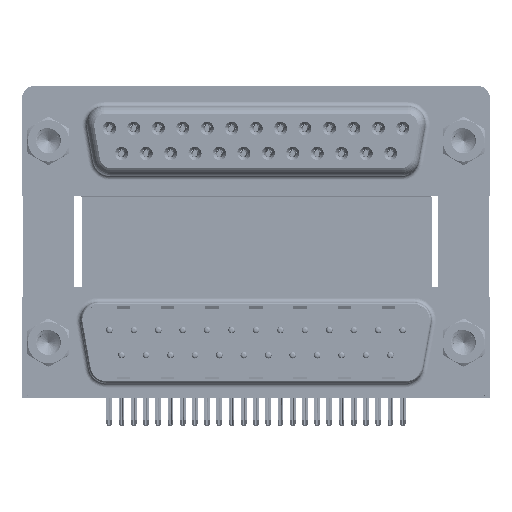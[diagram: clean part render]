
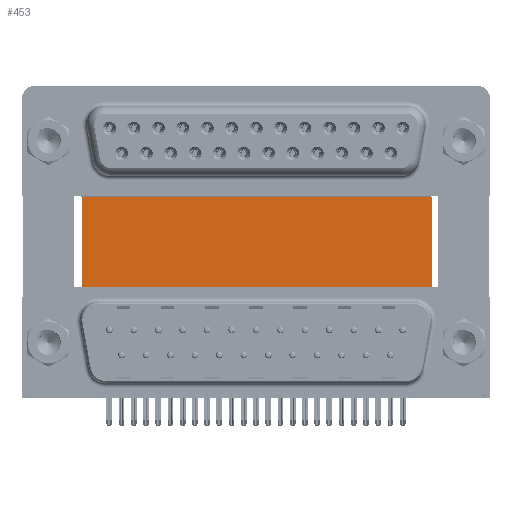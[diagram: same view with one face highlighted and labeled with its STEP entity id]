
A CAD part, top view. The second image highlights one B-rep face of the part: STEP entity #453.
In plain terms, the highlighted planar face has unit normal (0, 0, 1).
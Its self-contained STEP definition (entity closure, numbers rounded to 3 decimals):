
#93 = CARTESIAN_POINT ( 'NONE',  ( 3.79, 16.585, -12. ) ) ;
#308 = CARTESIAN_POINT ( 'NONE',  ( 43.43, 16.585, -12. ) ) ;
#453 = ADVANCED_FACE ( 'NONE', ( #34386 ), #1013, .F. ) ;
#1013 = PLANE ( 'NONE',  #60644 ) ;
#2868 = ORIENTED_EDGE ( 'NONE', *, *, #33222, .F. ) ;
#7323 = VERTEX_POINT ( 'NONE', #46095 ) ;
#10455 = DIRECTION ( 'NONE',  ( 0., 0., -1. ) ) ;
#12122 = VERTEX_POINT ( 'NONE', #308 ) ;
#15005 = LINE ( 'NONE', #48310, #37044 ) ;
#16457 = DIRECTION ( 'NONE',  ( 1., 0., 0. ) ) ;
#17712 = EDGE_CURVE ( 'NONE', #12122, #57683, #15005, .T. ) ;
#18959 = DIRECTION ( 'NONE',  ( 0., -1., 0. ) ) ;
#19459 = EDGE_CURVE ( 'NONE', #52430, #57683, #25617, .T. ) ;
#25617 = LINE ( 'NONE', #38851, #34199 ) ;
#25681 = VECTOR ( 'NONE', #16457, 1000. ) ;
#28084 = ORIENTED_EDGE ( 'NONE', *, *, #50141, .T. ) ;
#32612 = CARTESIAN_POINT ( 'NONE',  ( 3.79, -3.735, -12. ) ) ;
#33222 = EDGE_CURVE ( 'NONE', #7323, #12122, #40963, .T. ) ;
#33712 = LINE ( 'NONE', #53173, #38297 ) ;
#34198 = DIRECTION ( 'NONE',  ( 0., -1., 0. ) ) ;
#34199 = VECTOR ( 'NONE', #44788, 1000. ) ;
#34386 = FACE_OUTER_BOUND ( 'NONE', #46622, .T. ) ;
#37044 = VECTOR ( 'NONE', #34198, 1000. ) ;
#38297 = VECTOR ( 'NONE', #18959, 1000. ) ;
#38851 = CARTESIAN_POINT ( 'NONE',  ( 3.79, -3.735, -12. ) ) ;
#40963 = LINE ( 'NONE', #59491, #25681 ) ;
#44788 = DIRECTION ( 'NONE',  ( 1., 0., 0. ) ) ;
#46095 = CARTESIAN_POINT ( 'NONE',  ( 3.79, 16.585, -12. ) ) ;
#46622 = EDGE_LOOP ( 'NONE', ( #52943, #48992, #2868, #28084 ) ) ;
#48310 = CARTESIAN_POINT ( 'NONE',  ( 43.43, 16.585, -12. ) ) ;
#48992 = ORIENTED_EDGE ( 'NONE', *, *, #17712, .F. ) ;
#50141 = EDGE_CURVE ( 'NONE', #7323, #52430, #33712, .T. ) ;
#52430 = VERTEX_POINT ( 'NONE', #32612 ) ;
#52943 = ORIENTED_EDGE ( 'NONE', *, *, #19459, .T. ) ;
#53173 = CARTESIAN_POINT ( 'NONE',  ( 3.79, 16.585, -12. ) ) ;
#57620 = DIRECTION ( 'NONE',  ( -1., 0., 0. ) ) ;
#57683 = VERTEX_POINT ( 'NONE', #59091 ) ;
#59091 = CARTESIAN_POINT ( 'NONE',  ( 43.43, -3.735, -12. ) ) ;
#59491 = CARTESIAN_POINT ( 'NONE',  ( 3.79, 16.585, -12. ) ) ;
#60644 = AXIS2_PLACEMENT_3D ( 'NONE', #93, #10455, #57620 ) ;
